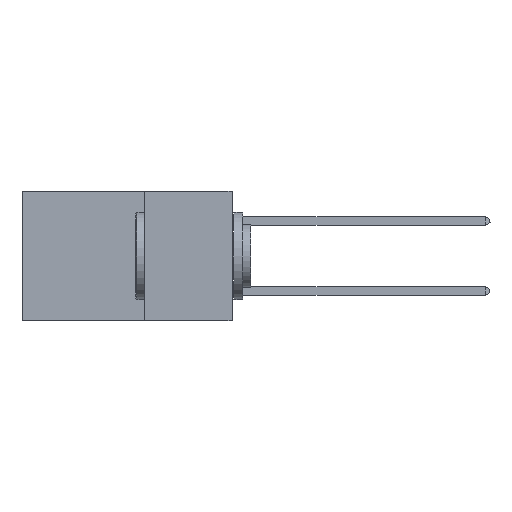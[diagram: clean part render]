
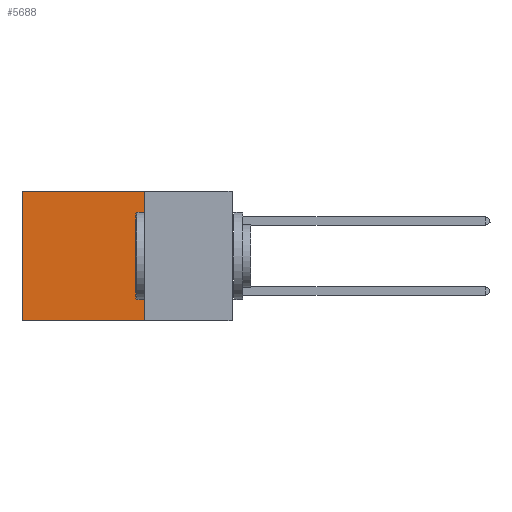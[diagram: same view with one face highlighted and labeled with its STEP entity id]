
A CAD part, left-side view. The second image highlights one B-rep face of the part: STEP entity #5688.
In plain terms, the highlighted planar face has unit normal (-1, 0, 0).
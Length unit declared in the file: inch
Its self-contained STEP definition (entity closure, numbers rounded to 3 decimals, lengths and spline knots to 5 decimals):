
#441 = DIRECTION ( 'NONE',  ( 0., 1., 0. ) ) ;
#1858 = VECTOR ( 'NONE', #7295, 39.37008 ) ;
#3613 = CARTESIAN_POINT ( 'NONE',  ( 0.2875, 0.25, -0.37 ) ) ;
#3967 = VECTOR ( 'NONE', #441, 39.37008 ) ;
#4963 = ORIENTED_EDGE ( 'NONE', *, *, #15713, .F. ) ;
#5169 = LINE ( 'NONE', #17488, #3967 ) ;
#5688 = ADVANCED_FACE ( 'NONE', ( #15307 ), #10056, .F. ) ;
#5765 = EDGE_CURVE ( 'NONE', #19799, #20957, #5169, .T. ) ;
#7295 = DIRECTION ( 'NONE',  ( 0., 1., 0. ) ) ;
#7429 = EDGE_LOOP ( 'NONE', ( #9767, #4963, #19025, #22920 ) ) ;
#7870 = VERTEX_POINT ( 'NONE', #18768 ) ;
#8167 = CARTESIAN_POINT ( 'NONE',  ( 0.2875, 0.6, 0. ) ) ;
#8398 = DIRECTION ( 'NONE',  ( 1., 0., 0. ) ) ;
#9554 = CARTESIAN_POINT ( 'NONE',  ( 0.2875, 0.25, 0. ) ) ;
#9767 = ORIENTED_EDGE ( 'NONE', *, *, #24063, .T. ) ;
#10056 = PLANE ( 'NONE',  #15659 ) ;
#12889 = LINE ( 'NONE', #22196, #1858 ) ;
#13435 = CARTESIAN_POINT ( 'NONE',  ( 0.2875, 0.6, 0. ) ) ;
#13761 = VECTOR ( 'NONE', #19071, 39.37008 ) ;
#14243 = LINE ( 'NONE', #13435, #23661 ) ;
#15307 = FACE_OUTER_BOUND ( 'NONE', #7429, .T. ) ;
#15659 = AXIS2_PLACEMENT_3D ( 'NONE', #17818, #8398, #16099 ) ;
#15713 = EDGE_CURVE ( 'NONE', #16274, #7870, #12889, .T. ) ;
#16099 = DIRECTION ( 'NONE',  ( 0., 0., -1. ) ) ;
#16274 = VERTEX_POINT ( 'NONE', #3613 ) ;
#17488 = CARTESIAN_POINT ( 'NONE',  ( 0.2875, 0.25, 0. ) ) ;
#17818 = CARTESIAN_POINT ( 'NONE',  ( 0.2875, 0.25, 0. ) ) ;
#18768 = CARTESIAN_POINT ( 'NONE',  ( 0.2875, 0.6, -0.37 ) ) ;
#18998 = CARTESIAN_POINT ( 'NONE',  ( 0.2875, 0.25, 0. ) ) ;
#19025 = ORIENTED_EDGE ( 'NONE', *, *, #22202, .F. ) ;
#19071 = DIRECTION ( 'NONE',  ( 0., 0., -1. ) ) ;
#19799 = VERTEX_POINT ( 'NONE', #18998 ) ;
#20740 = DIRECTION ( 'NONE',  ( 0., 0., -1. ) ) ;
#20957 = VERTEX_POINT ( 'NONE', #8167 ) ;
#22196 = CARTESIAN_POINT ( 'NONE',  ( 0.2875, 0.25, -0.37 ) ) ;
#22202 = EDGE_CURVE ( 'NONE', #19799, #16274, #23784, .T. ) ;
#22920 = ORIENTED_EDGE ( 'NONE', *, *, #5765, .T. ) ;
#23661 = VECTOR ( 'NONE', #20740, 39.37008 ) ;
#23784 = LINE ( 'NONE', #9554, #13761 ) ;
#24063 = EDGE_CURVE ( 'NONE', #20957, #7870, #14243, .T. ) ;
